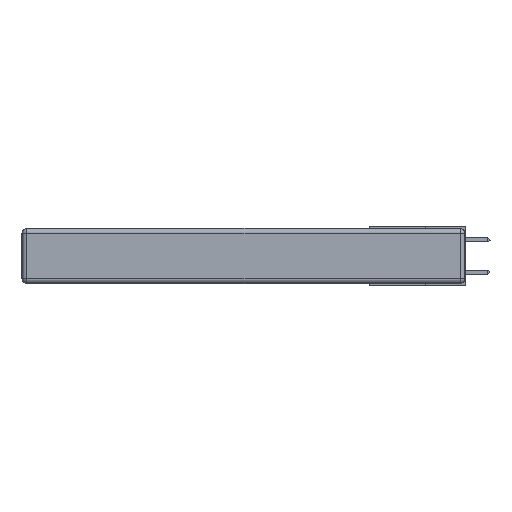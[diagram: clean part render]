
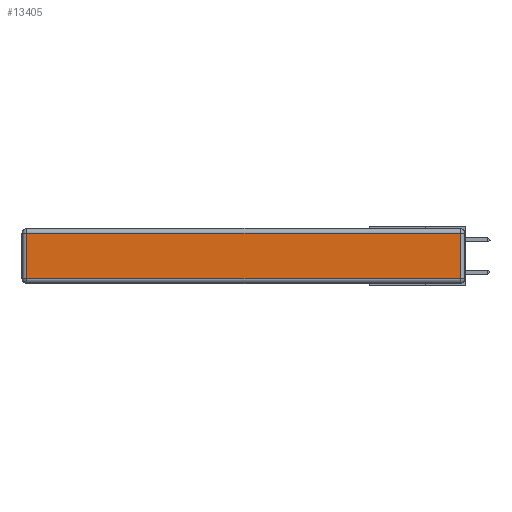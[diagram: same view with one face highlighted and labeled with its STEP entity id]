
A CAD part, left-side view. The second image highlights one B-rep face of the part: STEP entity #13405.
In plain terms, the highlighted planar face has unit normal (-1, 0, 0).
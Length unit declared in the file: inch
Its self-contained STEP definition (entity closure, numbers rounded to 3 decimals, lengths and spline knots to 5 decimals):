
#656 = EDGE_CURVE ( 'NONE', #4569, #7774, #5968, .T. ) ;
#875 = VECTOR ( 'NONE', #14539, 39.37008 ) ;
#2880 = VECTOR ( 'NONE', #17445, 39.37008 ) ;
#2912 = DIRECTION ( 'NONE',  ( 0., 0., 1. ) ) ;
#3728 = ORIENTED_EDGE ( 'NONE', *, *, #656, .T. ) ;
#3819 = FACE_OUTER_BOUND ( 'NONE', #9583, .T. ) ;
#4569 = VERTEX_POINT ( 'NONE', #11158 ) ;
#5928 = EDGE_CURVE ( 'NONE', #9788, #4569, #9956, .T. ) ;
#5968 = LINE ( 'NONE', #9474, #7811 ) ;
#6748 = VECTOR ( 'NONE', #14616, 39.37008 ) ;
#7468 = EDGE_CURVE ( 'NONE', #16082, #9788, #11733, .T. ) ;
#7774 = VERTEX_POINT ( 'NONE', #8320 ) ;
#7811 = VECTOR ( 'NONE', #11008, 39.37008 ) ;
#8039 = ORIENTED_EDGE ( 'NONE', *, *, #7468, .T. ) ;
#8320 = CARTESIAN_POINT ( 'NONE',  ( 0., 2.72, -0.03 ) ) ;
#8806 = DIRECTION ( 'NONE',  ( -1., 0., 0. ) ) ;
#9474 = CARTESIAN_POINT ( 'NONE',  ( 0., 2.75, -0.03 ) ) ;
#9583 = EDGE_LOOP ( 'NONE', ( #8039, #17247, #3728, #17343 ) ) ;
#9788 = VERTEX_POINT ( 'NONE', #19157 ) ;
#9956 = LINE ( 'NONE', #16327, #6748 ) ;
#9959 = CARTESIAN_POINT ( 'NONE',  ( 0., 0., -0.313 ) ) ;
#10774 = CARTESIAN_POINT ( 'NONE',  ( 0., 2.72, -0.313 ) ) ;
#11008 = DIRECTION ( 'NONE',  ( 0., 1., 0. ) ) ;
#11158 = CARTESIAN_POINT ( 'NONE',  ( 0., 0.03, -0.03 ) ) ;
#11538 = CARTESIAN_POINT ( 'NONE',  ( 0., 2.72, -0.343 ) ) ;
#11733 = LINE ( 'NONE', #9959, #875 ) ;
#13405 = ADVANCED_FACE ( 'NONE', ( #3819 ), #14670, .T. ) ;
#14539 = DIRECTION ( 'NONE',  ( 0., -1., 0. ) ) ;
#14616 = DIRECTION ( 'NONE',  ( 0., 0., 1. ) ) ;
#14670 = PLANE ( 'NONE',  #19060 ) ;
#15625 = LINE ( 'NONE', #11538, #2880 ) ;
#16082 = VERTEX_POINT ( 'NONE', #10774 ) ;
#16327 = CARTESIAN_POINT ( 'NONE',  ( 0., 0.03, -0.343 ) ) ;
#17247 = ORIENTED_EDGE ( 'NONE', *, *, #5928, .T. ) ;
#17343 = ORIENTED_EDGE ( 'NONE', *, *, #18138, .T. ) ;
#17445 = DIRECTION ( 'NONE',  ( 0., 0., -1. ) ) ;
#17809 = CARTESIAN_POINT ( 'NONE',  ( 0., 0., -0.343 ) ) ;
#18138 = EDGE_CURVE ( 'NONE', #7774, #16082, #15625, .T. ) ;
#19060 = AXIS2_PLACEMENT_3D ( 'NONE', #17809, #8806, #2912 ) ;
#19157 = CARTESIAN_POINT ( 'NONE',  ( 0., 0.03, -0.313 ) ) ;
